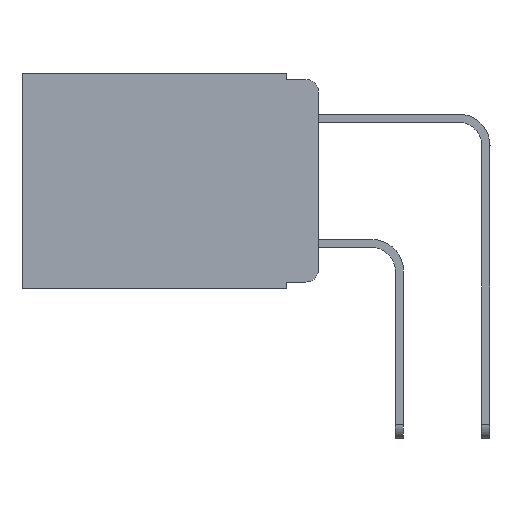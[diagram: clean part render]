
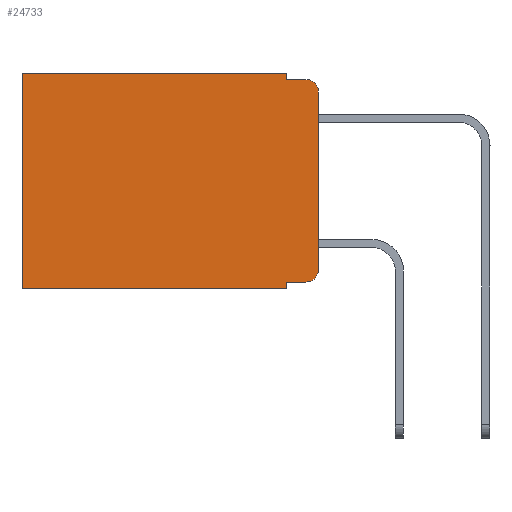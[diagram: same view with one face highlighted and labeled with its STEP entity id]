
A CAD part, left-side view. The second image highlights one B-rep face of the part: STEP entity #24733.
In plain terms, the highlighted planar face has unit normal (-1, 0, 0).
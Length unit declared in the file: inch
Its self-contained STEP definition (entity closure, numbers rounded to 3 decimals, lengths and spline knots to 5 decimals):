
#6 = CARTESIAN_POINT ( 'NONE',  ( 0.298, 0., 0. ) ) ;
#458 = CARTESIAN_POINT ( 'NONE',  ( 0.298, 0.051, -0.333 ) ) ;
#945 = VECTOR ( 'NONE', #3061, 39.37008 ) ;
#1358 = VERTEX_POINT ( 'NONE', #24742 ) ;
#1474 = EDGE_CURVE ( 'NONE', #11126, #24398, #26946, .T. ) ;
#2296 = DIRECTION ( 'NONE',  ( 0., 1., 0. ) ) ;
#2795 = CARTESIAN_POINT ( 'NONE',  ( 0.298, 0.02, -0.333 ) ) ;
#3061 = DIRECTION ( 'NONE',  ( 0., 0., -1. ) ) ;
#3543 = DIRECTION ( 'NONE',  ( 1., 0., 0. ) ) ;
#3548 = CARTESIAN_POINT ( 'NONE',  ( 0.298, 0.02, -0.313 ) ) ;
#3549 = CARTESIAN_POINT ( 'NONE',  ( 0.298, 0., 0. ) ) ;
#3773 = EDGE_CURVE ( 'NONE', #25617, #19701, #18346, .T. ) ;
#3829 = DIRECTION ( 'NONE',  ( 0., 0., -1. ) ) ;
#4396 = EDGE_CURVE ( 'NONE', #1358, #21927, #22260, .T. ) ;
#4737 = LINE ( 'NONE', #3549, #16829 ) ;
#5064 = VECTOR ( 'NONE', #20631, 39.37008 ) ;
#5616 = VECTOR ( 'NONE', #25167, 39.37008 ) ;
#7137 = ORIENTED_EDGE ( 'NONE', *, *, #16333, .T. ) ;
#7511 = ORIENTED_EDGE ( 'NONE', *, *, #21842, .F. ) ;
#7921 = CIRCLE ( 'NONE', #13988, 0.02 ) ;
#8774 = VERTEX_POINT ( 'NONE', #2795 ) ;
#9596 = CARTESIAN_POINT ( 'NONE',  ( 0.298, 0., -0.313 ) ) ;
#10148 = EDGE_CURVE ( 'NONE', #25617, #19649, #4737, .T. ) ;
#10402 = CARTESIAN_POINT ( 'NONE',  ( 0.298, 0.051, 0. ) ) ;
#10552 = AXIS2_PLACEMENT_3D ( 'NONE', #26712, #3543, #20328 ) ;
#10710 = EDGE_CURVE ( 'NONE', #24398, #18629, #15168, .T. ) ;
#11126 = VERTEX_POINT ( 'NONE', #458 ) ;
#11775 = CARTESIAN_POINT ( 'NONE',  ( 0.298, 0.02, -0.01 ) ) ;
#12028 = LINE ( 'NONE', #23936, #945 ) ;
#12105 = PLANE ( 'NONE',  #10552 ) ;
#12704 = CARTESIAN_POINT ( 'NONE',  ( 0.298, 0., -0.03 ) ) ;
#12995 = CARTESIAN_POINT ( 'NONE',  ( 0.298, 0.051, -0.333 ) ) ;
#13076 = DIRECTION ( 'NONE',  ( 0., -1., 0. ) ) ;
#13910 = EDGE_CURVE ( 'NONE', #19367, #18629, #12028, .T. ) ;
#13988 = AXIS2_PLACEMENT_3D ( 'NONE', #3548, #20241, #20072 ) ;
#14155 = DIRECTION ( 'NONE',  ( -1., 0., 0. ) ) ;
#14867 = ORIENTED_EDGE ( 'NONE', *, *, #10148, .F. ) ;
#14891 = LINE ( 'NONE', #12995, #21086 ) ;
#15168 = LINE ( 'NONE', #23216, #19408 ) ;
#15322 = CARTESIAN_POINT ( 'NONE',  ( 0.298, 0.051, -0.01 ) ) ;
#15450 = ORIENTED_EDGE ( 'NONE', *, *, #3773, .T. ) ;
#16237 = EDGE_LOOP ( 'NONE', ( #14867, #15450, #7511, #22624, #20347, #21021, #23284, #23231, #7137, #23617 ) ) ;
#16247 = DIRECTION ( 'NONE',  ( 0., 0., -1. ) ) ;
#16333 = EDGE_CURVE ( 'NONE', #11126, #8774, #14891, .T. ) ;
#16829 = VECTOR ( 'NONE', #3829, 39.37008 ) ;
#17060 = CARTESIAN_POINT ( 'NONE',  ( 0.298, 0.051, -0.01 ) ) ;
#17194 = CARTESIAN_POINT ( 'NONE',  ( 0.298, 0.473, -0.343 ) ) ;
#17519 = VECTOR ( 'NONE', #21161, 39.37008 ) ;
#18201 = VECTOR ( 'NONE', #2296, 39.37008 ) ;
#18346 = CIRCLE ( 'NONE', #24472, 0.02 ) ;
#18430 = EDGE_CURVE ( 'NONE', #8774, #19649, #7921, .T. ) ;
#18476 = CARTESIAN_POINT ( 'NONE',  ( 0.298, 0.02, -0.03 ) ) ;
#18629 = VERTEX_POINT ( 'NONE', #17194 ) ;
#18898 = CARTESIAN_POINT ( 'NONE',  ( 0.298, 0.051, 0. ) ) ;
#19367 = VERTEX_POINT ( 'NONE', #25407 ) ;
#19408 = VECTOR ( 'NONE', #26742, 39.37008 ) ;
#19649 = VERTEX_POINT ( 'NONE', #9596 ) ;
#19701 = VERTEX_POINT ( 'NONE', #11775 ) ;
#20072 = DIRECTION ( 'NONE',  ( 0., 0., -1. ) ) ;
#20241 = DIRECTION ( 'NONE',  ( -1., 0., 0. ) ) ;
#20328 = DIRECTION ( 'NONE',  ( 0., 0., -1. ) ) ;
#20347 = ORIENTED_EDGE ( 'NONE', *, *, #21767, .T. ) ;
#20631 = DIRECTION ( 'NONE',  ( 0., 0., -1. ) ) ;
#21021 = ORIENTED_EDGE ( 'NONE', *, *, #13910, .T. ) ;
#21086 = VECTOR ( 'NONE', #13076, 39.37008 ) ;
#21161 = DIRECTION ( 'NONE',  ( 0., -1., 0. ) ) ;
#21767 = EDGE_CURVE ( 'NONE', #1358, #19367, #23702, .T. ) ;
#21835 = FACE_OUTER_BOUND ( 'NONE', #16237, .T. ) ;
#21842 = EDGE_CURVE ( 'NONE', #21927, #19701, #25042, .T. ) ;
#21927 = VERTEX_POINT ( 'NONE', #15322 ) ;
#22260 = LINE ( 'NONE', #18898, #5616 ) ;
#22624 = ORIENTED_EDGE ( 'NONE', *, *, #4396, .F. ) ;
#23216 = CARTESIAN_POINT ( 'NONE',  ( 0.298, 0., -0.343 ) ) ;
#23231 = ORIENTED_EDGE ( 'NONE', *, *, #1474, .F. ) ;
#23284 = ORIENTED_EDGE ( 'NONE', *, *, #10710, .F. ) ;
#23503 = CARTESIAN_POINT ( 'NONE',  ( 0.298, 0.051, -0.343 ) ) ;
#23617 = ORIENTED_EDGE ( 'NONE', *, *, #18430, .T. ) ;
#23702 = LINE ( 'NONE', #6, #18201 ) ;
#23936 = CARTESIAN_POINT ( 'NONE',  ( 0.298, 0.473, 0. ) ) ;
#24398 = VERTEX_POINT ( 'NONE', #23503 ) ;
#24472 = AXIS2_PLACEMENT_3D ( 'NONE', #18476, #14155, #16247 ) ;
#24733 = ADVANCED_FACE ( 'NONE', ( #21835 ), #12105, .F. ) ;
#24742 = CARTESIAN_POINT ( 'NONE',  ( 0.298, 0.051, 0. ) ) ;
#25042 = LINE ( 'NONE', #17060, #17519 ) ;
#25167 = DIRECTION ( 'NONE',  ( 0., 0., -1. ) ) ;
#25407 = CARTESIAN_POINT ( 'NONE',  ( 0.298, 0.473, 0. ) ) ;
#25617 = VERTEX_POINT ( 'NONE', #12704 ) ;
#26712 = CARTESIAN_POINT ( 'NONE',  ( 0.298, 0., 0. ) ) ;
#26742 = DIRECTION ( 'NONE',  ( 0., 1., 0. ) ) ;
#26946 = LINE ( 'NONE', #10402, #5064 ) ;
